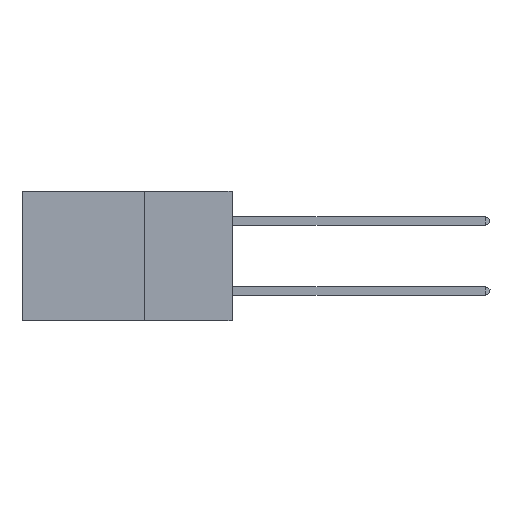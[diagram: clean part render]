
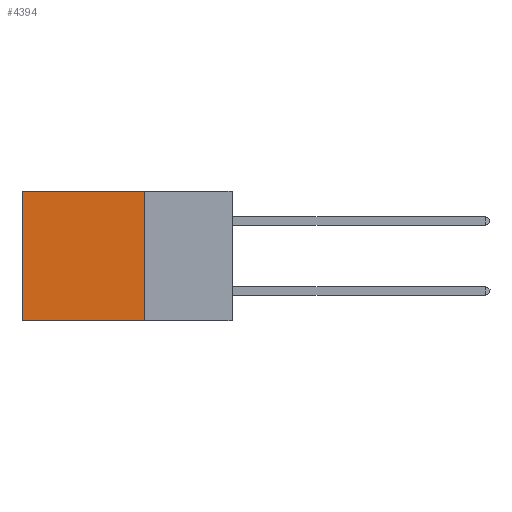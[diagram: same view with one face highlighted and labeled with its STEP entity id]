
A CAD part, left-side view. The second image highlights one B-rep face of the part: STEP entity #4394.
In plain terms, the highlighted planar face has unit normal (-1, 0, 0).
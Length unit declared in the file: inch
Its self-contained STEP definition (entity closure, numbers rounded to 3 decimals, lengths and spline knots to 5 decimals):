
#98 = CARTESIAN_POINT ( 'NONE',  ( 0.2875, 0.25, 0. ) ) ;
#349 = DIRECTION ( 'NONE',  ( 0., 1., 0. ) ) ;
#550 = CARTESIAN_POINT ( 'NONE',  ( 0.2875, 0.25, 0. ) ) ;
#631 = VERTEX_POINT ( 'NONE', #3992 ) ;
#1027 = LINE ( 'NONE', #550, #12239 ) ;
#1332 = EDGE_LOOP ( 'NONE', ( #12618, #9890, #4202, #14400 ) ) ;
#1615 = CARTESIAN_POINT ( 'NONE',  ( 0.2875, 0.6, 0. ) ) ;
#3418 = AXIS2_PLACEMENT_3D ( 'NONE', #11911, #15597, #12934 ) ;
#3430 = VECTOR ( 'NONE', #11375, 39.37008 ) ;
#3557 = VECTOR ( 'NONE', #349, 39.37008 ) ;
#3864 = LINE ( 'NONE', #98, #3557 ) ;
#3989 = FACE_OUTER_BOUND ( 'NONE', #1332, .T. ) ;
#3992 = CARTESIAN_POINT ( 'NONE',  ( 0.2875, 0.25, -0.37 ) ) ;
#4202 = ORIENTED_EDGE ( 'NONE', *, *, #4516, .F. ) ;
#4268 = VERTEX_POINT ( 'NONE', #7483 ) ;
#4394 = ADVANCED_FACE ( 'NONE', ( #3989 ), #15346, .F. ) ;
#4516 = EDGE_CURVE ( 'NONE', #4268, #631, #1027, .T. ) ;
#4531 = CARTESIAN_POINT ( 'NONE',  ( 0.2875, 0.25, -0.37 ) ) ;
#4652 = EDGE_CURVE ( 'NONE', #13229, #6869, #15478, .T. ) ;
#6869 = VERTEX_POINT ( 'NONE', #15776 ) ;
#7483 = CARTESIAN_POINT ( 'NONE',  ( 0.2875, 0.25, 0. ) ) ;
#7725 = EDGE_CURVE ( 'NONE', #4268, #13229, #3864, .T. ) ;
#8886 = VECTOR ( 'NONE', #15727, 39.37008 ) ;
#9890 = ORIENTED_EDGE ( 'NONE', *, *, #10202, .F. ) ;
#10202 = EDGE_CURVE ( 'NONE', #631, #6869, #13559, .T. ) ;
#10806 = DIRECTION ( 'NONE',  ( 0., 0., -1. ) ) ;
#11375 = DIRECTION ( 'NONE',  ( 0., 0., -1. ) ) ;
#11911 = CARTESIAN_POINT ( 'NONE',  ( 0.2875, 0.25, 0. ) ) ;
#12239 = VECTOR ( 'NONE', #10806, 39.37008 ) ;
#12618 = ORIENTED_EDGE ( 'NONE', *, *, #4652, .T. ) ;
#12646 = CARTESIAN_POINT ( 'NONE',  ( 0.2875, 0.6, 0. ) ) ;
#12934 = DIRECTION ( 'NONE',  ( 0., 0., -1. ) ) ;
#13229 = VERTEX_POINT ( 'NONE', #1615 ) ;
#13559 = LINE ( 'NONE', #4531, #8886 ) ;
#14400 = ORIENTED_EDGE ( 'NONE', *, *, #7725, .T. ) ;
#15346 = PLANE ( 'NONE',  #3418 ) ;
#15478 = LINE ( 'NONE', #12646, #3430 ) ;
#15597 = DIRECTION ( 'NONE',  ( 1., 0., 0. ) ) ;
#15727 = DIRECTION ( 'NONE',  ( 0., 1., 0. ) ) ;
#15776 = CARTESIAN_POINT ( 'NONE',  ( 0.2875, 0.6, -0.37 ) ) ;
